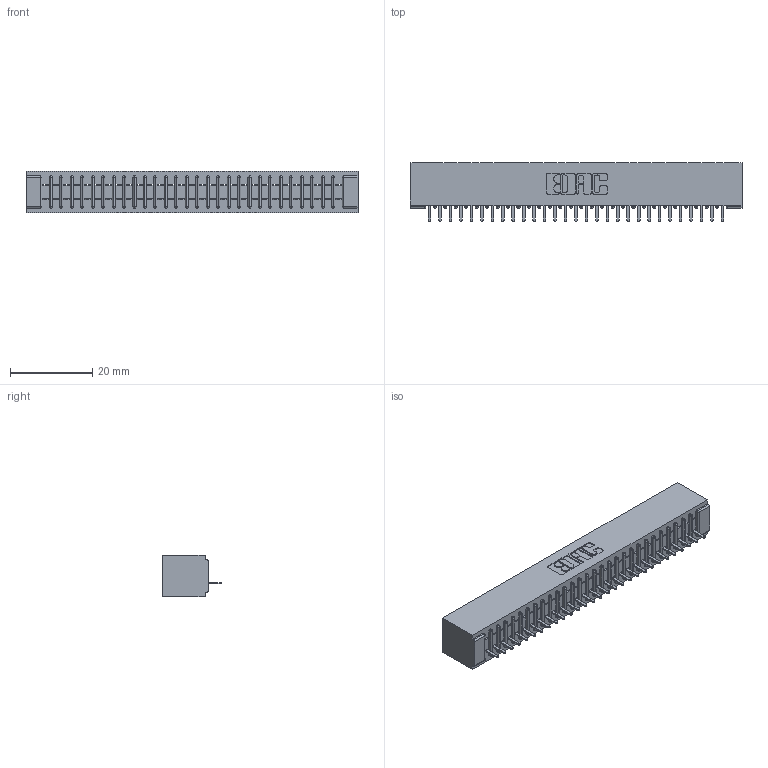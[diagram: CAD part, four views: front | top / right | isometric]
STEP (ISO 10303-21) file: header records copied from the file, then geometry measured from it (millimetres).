
FILE_DESCRIPTION (( 'STEP AP203' ), '1' );
FILE_NAME ('341-029-520-101.STEP', '2018-08-06T19:42:26', ( '' ), ( '' ), 'SwSTEP 2.0', 'SolidWorks 2016', '' );
FILE_SCHEMA (( 'CONFIG_CONTROL_DESIGN' ));
Length unit declared in the file: inch
Products named in the file (3): 341-292-001_341-292-120; 341-029-520-101; 341 Part_No Mounting Lugs
Assembly tree (30 placements, depth 2):
  341-029-520-101
    341 Part_No Mounting Lugs
    341-292-001_341-292-120  x29
Bounding box: 80.64 x 14.27 x 10.16 mm (x, y, z)
Volume: 5973.2 mm3; surface area: 9383.7 mm2
Topology: 30 solids, 30 shells, 2486 faces, 7165 edges, 4598 vertices
Faces by surface type: plane 1543, cylinder 827, sphere 60, torus 56
Entity records: 35622 total; most frequent: CARTESIAN_POINT 6046, ORIENTED_EDGE 6034, DIRECTION 5845, EDGE_CURVE 3017, LINE 2427, VECTOR 2427, VERTEX_POINT 1910, AXIS2_PLACEMENT_3D 1709
